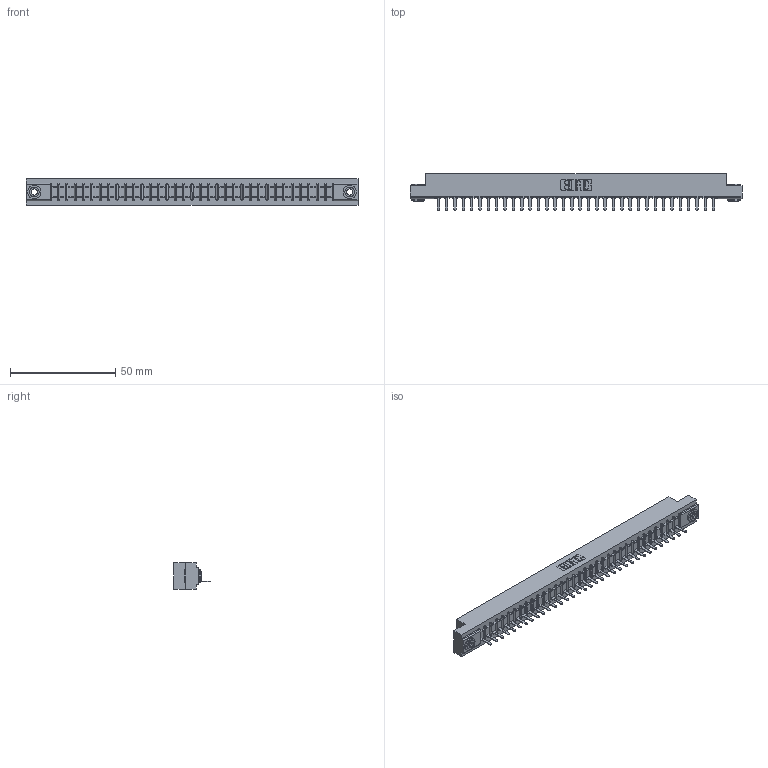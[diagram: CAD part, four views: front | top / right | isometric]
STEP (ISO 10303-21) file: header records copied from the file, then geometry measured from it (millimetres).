
FILE_DESCRIPTION (( 'STEP AP203' ), '1' );
FILE_NAME ('357-034-421-103.STEP', '2020-10-02T10:29:25', ( '' ), ( '' ), 'SwSTEP 2.0', 'SolidWorks 2020', '' );
FILE_SCHEMA (( 'CONFIG_CONTROL_DESIGN' ));
Length unit declared in the file: inch
Products named in the file (4): 345-250-002_345-250-002-102; 357-034-421-103; 307 Part_.156 Dia Mounting Holes; 307-290-002_521
Assembly tree (37 placements, depth 2):
  357-034-421-103
    307 Part_.156 Dia Mounting Holes
    307-290-002_521  x34
    345-250-002_345-250-002-102  x2
Bounding box: 157.73 x 17.42 x 12.7 mm (x, y, z)
Volume: 16823.2 mm3; surface area: 21232.5 mm2
Topology: 37 solids, 37 shells, 2721 faces, 8323 edges, 5450 vertices
Faces by surface type: plane 1624, cylinder 1019, sphere 70, cone 8
Entity records: 31917 total; most frequent: CARTESIAN_POINT 5361, ORIENTED_EDGE 5342, DIRECTION 5227, EDGE_CURVE 2671, VECTOR 2035, LINE 2035, VERTEX_POINT 1730, AXIS2_PLACEMENT_3D 1596
